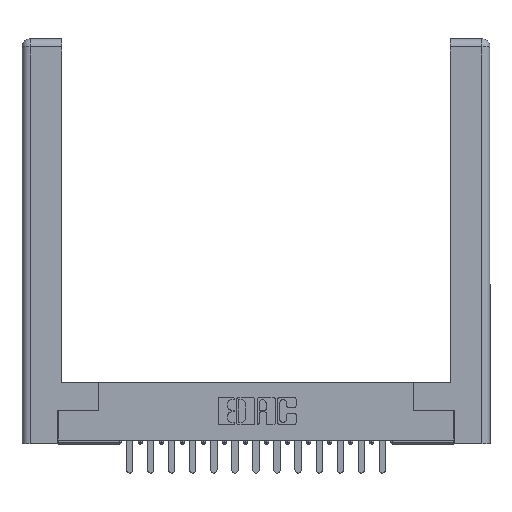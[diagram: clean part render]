
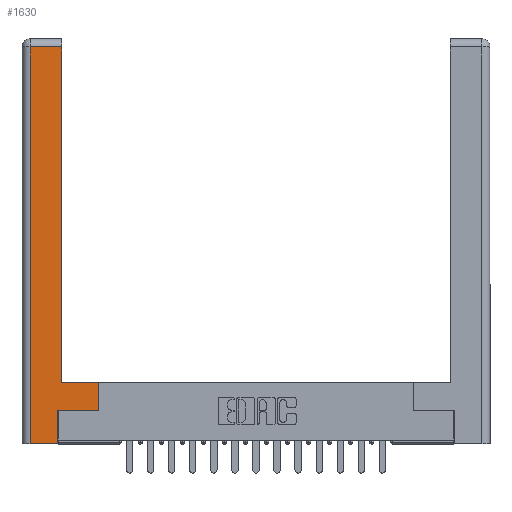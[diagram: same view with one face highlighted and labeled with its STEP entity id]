
A CAD part, top view. The second image highlights one B-rep face of the part: STEP entity #1630.
In plain terms, the highlighted planar face has unit normal (0, 0, 1).
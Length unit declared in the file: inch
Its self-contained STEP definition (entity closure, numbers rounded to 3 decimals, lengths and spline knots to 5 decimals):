
#164 = VERTEX_POINT ( 'NONE', #2533 ) ;
#558 = CARTESIAN_POINT ( 'NONE',  ( 0.295, 2.94, 0. ) ) ;
#642 = DIRECTION ( 'NONE',  ( -1., 0., 0. ) ) ;
#1601 = VECTOR ( 'NONE', #12722, 39.37008 ) ;
#1614 = CARTESIAN_POINT ( 'NONE',  ( 0.265, 0.245, 0. ) ) ;
#1630 = ADVANCED_FACE ( 'NONE', ( #8944 ), #7635, .F. ) ;
#2240 = DIRECTION ( 'NONE',  ( 1., 0., 0. ) ) ;
#2351 = CARTESIAN_POINT ( 'NONE',  ( 0.295, 0.45, 0. ) ) ;
#2533 = CARTESIAN_POINT ( 'NONE',  ( 0.295, 0.45, 0. ) ) ;
#2609 = VERTEX_POINT ( 'NONE', #7095 ) ;
#2834 = ORIENTED_EDGE ( 'NONE', *, *, #13977, .T. ) ;
#2964 = CARTESIAN_POINT ( 'NONE',  ( 0.565, 0.45, 0. ) ) ;
#2991 = EDGE_CURVE ( 'NONE', #13629, #7283, #16993, .T. ) ;
#3055 = ORIENTED_EDGE ( 'NONE', *, *, #10844, .T. ) ;
#3226 = CARTESIAN_POINT ( 'NONE',  ( 0.265, 0., 0. ) ) ;
#3553 = LINE ( 'NONE', #2351, #13211 ) ;
#3873 = LINE ( 'NONE', #9568, #5159 ) ;
#4145 = CARTESIAN_POINT ( 'NONE',  ( 0.265, 0., 0. ) ) ;
#4249 = ORIENTED_EDGE ( 'NONE', *, *, #13749, .T. ) ;
#4282 = CARTESIAN_POINT ( 'NONE',  ( 0.0615, 0., 0. ) ) ;
#4858 = CARTESIAN_POINT ( 'NONE',  ( 0., 0., 0. ) ) ;
#4891 = VERTEX_POINT ( 'NONE', #3226 ) ;
#5159 = VECTOR ( 'NONE', #13877, 39.37008 ) ;
#5438 = CARTESIAN_POINT ( 'NONE',  ( 0.0615, 0., 0. ) ) ;
#5592 = DIRECTION ( 'NONE',  ( 0., -1., 0. ) ) ;
#5677 = LINE ( 'NONE', #7156, #17313 ) ;
#6039 = CARTESIAN_POINT ( 'NONE',  ( 0.565, 0.245, 0. ) ) ;
#6531 = ORIENTED_EDGE ( 'NONE', *, *, #7643, .T. ) ;
#6536 = CARTESIAN_POINT ( 'NONE',  ( 0.0615, 2.94, 0. ) ) ;
#6614 = CARTESIAN_POINT ( 'NONE',  ( 0.565, 0.245, 0. ) ) ;
#6933 = LINE ( 'NONE', #1614, #1601 ) ;
#7095 = CARTESIAN_POINT ( 'NONE',  ( 0.265, 0.245, 0. ) ) ;
#7125 = LINE ( 'NONE', #4145, #15778 ) ;
#7156 = CARTESIAN_POINT ( 'NONE',  ( 0.295, 3., 0. ) ) ;
#7283 = VERTEX_POINT ( 'NONE', #5438 ) ;
#7635 = PLANE ( 'NONE',  #12453 ) ;
#7640 = EDGE_LOOP ( 'NONE', ( #13172, #2834, #15863, #3055, #4249, #6531, #15163, #11756 ) ) ;
#7643 = EDGE_CURVE ( 'NONE', #2609, #15071, #15401, .T. ) ;
#8944 = FACE_OUTER_BOUND ( 'NONE', #7640, .T. ) ;
#9162 = EDGE_CURVE ( 'NONE', #164, #14651, #5677, .T. ) ;
#9319 = DIRECTION ( 'NONE',  ( 0., 0., -1. ) ) ;
#9568 = CARTESIAN_POINT ( 'NONE',  ( 0.565, 0.45, 0. ) ) ;
#10534 = VECTOR ( 'NONE', #13832, 39.37008 ) ;
#10844 = EDGE_CURVE ( 'NONE', #7283, #4891, #7125, .T. ) ;
#11372 = DIRECTION ( 'NONE',  ( 0., 1., 0. ) ) ;
#11756 = ORIENTED_EDGE ( 'NONE', *, *, #14045, .T. ) ;
#12129 = VECTOR ( 'NONE', #5592, 39.37008 ) ;
#12453 = AXIS2_PLACEMENT_3D ( 'NONE', #4858, #9319, #642 ) ;
#12722 = DIRECTION ( 'NONE',  ( 0., 1., 0. ) ) ;
#12822 = DIRECTION ( 'NONE',  ( 1., 0., 0. ) ) ;
#13172 = ORIENTED_EDGE ( 'NONE', *, *, #9162, .T. ) ;
#13211 = VECTOR ( 'NONE', #17784, 39.37008 ) ;
#13262 = EDGE_CURVE ( 'NONE', #15071, #14865, #3873, .T. ) ;
#13629 = VERTEX_POINT ( 'NONE', #13666 ) ;
#13666 = CARTESIAN_POINT ( 'NONE',  ( 0.0615, 2.94, 0. ) ) ;
#13749 = EDGE_CURVE ( 'NONE', #4891, #2609, #6933, .T. ) ;
#13832 = DIRECTION ( 'NONE',  ( -1., 0., 0. ) ) ;
#13877 = DIRECTION ( 'NONE',  ( 0., 1., 0. ) ) ;
#13977 = EDGE_CURVE ( 'NONE', #14651, #13629, #16639, .T. ) ;
#14045 = EDGE_CURVE ( 'NONE', #14865, #164, #3553, .T. ) ;
#14651 = VERTEX_POINT ( 'NONE', #558 ) ;
#14865 = VERTEX_POINT ( 'NONE', #2964 ) ;
#15071 = VERTEX_POINT ( 'NONE', #6039 ) ;
#15163 = ORIENTED_EDGE ( 'NONE', *, *, #13262, .T. ) ;
#15401 = LINE ( 'NONE', #6614, #17986 ) ;
#15778 = VECTOR ( 'NONE', #12822, 39.37008 ) ;
#15863 = ORIENTED_EDGE ( 'NONE', *, *, #2991, .T. ) ;
#16639 = LINE ( 'NONE', #6536, #10534 ) ;
#16993 = LINE ( 'NONE', #4282, #12129 ) ;
#17313 = VECTOR ( 'NONE', #11372, 39.37008 ) ;
#17784 = DIRECTION ( 'NONE',  ( -1., 0., 0. ) ) ;
#17986 = VECTOR ( 'NONE', #2240, 39.37008 ) ;
